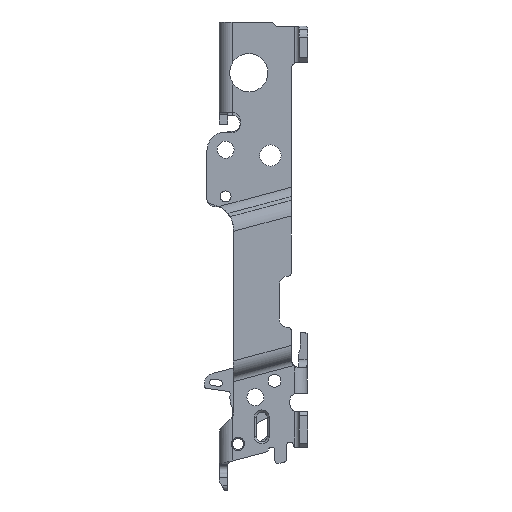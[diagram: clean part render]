
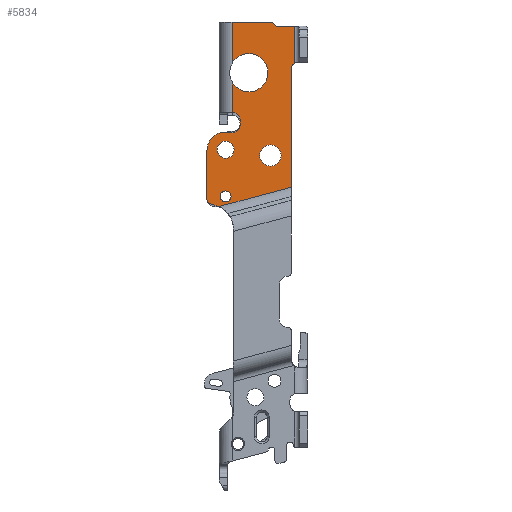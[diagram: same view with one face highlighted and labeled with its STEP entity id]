
A CAD part, left-side view. The second image highlights one B-rep face of the part: STEP entity #5834.
In plain terms, the highlighted planar face has unit normal (-1, 0, 0).
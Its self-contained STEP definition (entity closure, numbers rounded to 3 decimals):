
#43=FACE_BOUND('',#762,.T.);
#44=FACE_BOUND('',#763,.T.);
#45=FACE_BOUND('',#764,.T.);
#209=PLANE('',#6303);
#427=FACE_OUTER_BOUND('',#761,.T.);
#761=EDGE_LOOP('',(#4413,#4414,#4415,#4416,#4417,#4418,#4419,#4420,#4421,
#4422,#4423,#4424,#4425,#4426,#4427,#4428,#4429,#4430,#4431,#4432));
#762=EDGE_LOOP('',(#4433));
#763=EDGE_LOOP('',(#4434));
#764=EDGE_LOOP('',(#4435));
#1129=LINE('',#8839,#1689);
#1133=LINE('',#8849,#1693);
#1139=LINE('',#8872,#1699);
#1140=LINE('',#8874,#1700);
#1215=LINE('',#9234,#1775);
#1237=LINE('',#9377,#1797);
#1238=LINE('',#9381,#1798);
#1239=LINE('',#9384,#1799);
#1240=LINE('',#9386,#1800);
#1241=LINE('',#9388,#1801);
#1242=LINE('',#9390,#1802);
#1243=LINE('',#9392,#1803);
#1244=LINE('',#9393,#1804);
#1689=VECTOR('',#7012,10.);
#1693=VECTOR('',#7024,10.);
#1699=VECTOR('',#7040,10.);
#1700=VECTOR('',#7041,10.);
#1775=VECTOR('',#7314,10.);
#1797=VECTOR('',#7374,10.);
#1798=VECTOR('',#7377,10.);
#1799=VECTOR('',#7380,10.);
#1800=VECTOR('',#7381,10.);
#1801=VECTOR('',#7382,10.);
#1802=VECTOR('',#7383,10.);
#1803=VECTOR('',#7384,10.);
#1804=VECTOR('',#7385,10.);
#2129=CIRCLE('',#6093,2.);
#2173=CIRCLE('',#6180,2.);
#2186=CIRCLE('',#6208,2.);
#2222=CIRCLE('',#6261,2.5);
#2223=CIRCLE('',#6264,1.275);
#2227=CIRCLE('',#6272,4.5);
#2235=CIRCLE('',#6302,1.5);
#2236=CIRCLE('',#6304,4.5);
#2237=CIRCLE('',#6305,1.);
#2238=CIRCLE('',#6306,6.);
#2382=VERTEX_POINT('',#8486);
#2384=VERTEX_POINT('',#8490);
#2385=VERTEX_POINT('',#8494);
#2388=VERTEX_POINT('',#8508);
#2510=VERTEX_POINT('',#8836);
#2511=VERTEX_POINT('',#8838);
#2513=VERTEX_POINT('',#8844);
#2518=VERTEX_POINT('',#8873);
#2534=VERTEX_POINT('',#8996);
#2601=VERTEX_POINT('',#9171);
#2602=VERTEX_POINT('',#9177);
#2610=VERTEX_POINT('',#9231);
#2611=VERTEX_POINT('',#9233);
#2638=VERTEX_POINT('',#9368);
#2640=VERTEX_POINT('',#9374);
#2641=VERTEX_POINT('',#9376);
#2642=VERTEX_POINT('',#9378);
#2643=VERTEX_POINT('',#9380);
#2644=VERTEX_POINT('',#9382);
#2645=VERTEX_POINT('',#9385);
#2646=VERTEX_POINT('',#9387);
#2647=VERTEX_POINT('',#9389);
#2648=VERTEX_POINT('',#9391);
#2960=EDGE_CURVE('',#2382,#2384,#2129,.T.);
#3120=EDGE_CURVE('',#2511,#2510,#1129,.T.);
#3123=EDGE_CURVE('',#2513,#2511,#2173,.T.);
#3126=EDGE_CURVE('',#2384,#2513,#1133,.T.);
#3136=EDGE_CURVE('',#2385,#2382,#1139,.T.);
#3137=EDGE_CURVE('',#2518,#2388,#1140,.T.);
#3166=EDGE_CURVE('',#2534,#2534,#2186,.T.);
#3257=EDGE_CURVE('',#2601,#2601,#2222,.T.);
#3260=EDGE_CURVE('',#2602,#2602,#2223,.T.);
#3267=EDGE_CURVE('',#2388,#2385,#2227,.T.);
#3279=EDGE_CURVE('',#2611,#2610,#1215,.T.);
#3315=EDGE_CURVE('',#2638,#2610,#2235,.T.);
#3317=EDGE_CURVE('',#2510,#2640,#2236,.T.);
#3318=EDGE_CURVE('',#2640,#2641,#1237,.T.);
#3319=EDGE_CURVE('',#2641,#2642,#2237,.T.);
#3320=EDGE_CURVE('',#2642,#2643,#1238,.T.);
#3321=EDGE_CURVE('',#2643,#2644,#2238,.T.);
#3322=EDGE_CURVE('',#2644,#2611,#1239,.T.);
#3323=EDGE_CURVE('',#2645,#2638,#1240,.T.);
#3324=EDGE_CURVE('',#2645,#2646,#1241,.T.);
#3325=EDGE_CURVE('',#2647,#2646,#1242,.T.);
#3326=EDGE_CURVE('',#2647,#2648,#1243,.T.);
#3327=EDGE_CURVE('',#2648,#2518,#1244,.T.);
#4413=ORIENTED_EDGE('',*,*,#3120,.T.);
#4414=ORIENTED_EDGE('',*,*,#3317,.T.);
#4415=ORIENTED_EDGE('',*,*,#3318,.T.);
#4416=ORIENTED_EDGE('',*,*,#3319,.T.);
#4417=ORIENTED_EDGE('',*,*,#3320,.T.);
#4418=ORIENTED_EDGE('',*,*,#3321,.T.);
#4419=ORIENTED_EDGE('',*,*,#3322,.T.);
#4420=ORIENTED_EDGE('',*,*,#3279,.T.);
#4421=ORIENTED_EDGE('',*,*,#3315,.F.);
#4422=ORIENTED_EDGE('',*,*,#3323,.F.);
#4423=ORIENTED_EDGE('',*,*,#3324,.T.);
#4424=ORIENTED_EDGE('',*,*,#3325,.F.);
#4425=ORIENTED_EDGE('',*,*,#3326,.T.);
#4426=ORIENTED_EDGE('',*,*,#3327,.T.);
#4427=ORIENTED_EDGE('',*,*,#3137,.T.);
#4428=ORIENTED_EDGE('',*,*,#3267,.T.);
#4429=ORIENTED_EDGE('',*,*,#3136,.T.);
#4430=ORIENTED_EDGE('',*,*,#2960,.T.);
#4431=ORIENTED_EDGE('',*,*,#3126,.T.);
#4432=ORIENTED_EDGE('',*,*,#3123,.T.);
#4433=ORIENTED_EDGE('',*,*,#3257,.T.);
#4434=ORIENTED_EDGE('',*,*,#3260,.T.);
#4435=ORIENTED_EDGE('',*,*,#3166,.T.);
#5834=ADVANCED_FACE('',(#427,#43,#44,#45),#209,.T.);
#6093=AXIS2_PLACEMENT_3D('',#8492,#6733,#6734);
#6180=AXIS2_PLACEMENT_3D('',#8845,#7018,#7019);
#6208=AXIS2_PLACEMENT_3D('',#8998,#7093,#7094);
#6261=AXIS2_PLACEMENT_3D('',#9173,#7254,#7255);
#6264=AXIS2_PLACEMENT_3D('',#9179,#7262,#7263);
#6272=AXIS2_PLACEMENT_3D('',#9193,#7281,#7282);
#6302=AXIS2_PLACEMENT_3D('',#9371,#7367,#7368);
#6303=AXIS2_PLACEMENT_3D('',#9373,#7370,#7371);
#6304=AXIS2_PLACEMENT_3D('',#9375,#7372,#7373);
#6305=AXIS2_PLACEMENT_3D('',#9379,#7375,#7376);
#6306=AXIS2_PLACEMENT_3D('',#9383,#7378,#7379);
#6733=DIRECTION('center_axis',(1.,0.,0.));
#6734=DIRECTION('ref_axis',(0.,-1.,0.));
#7012=DIRECTION('',(0.,1.,0.));
#7018=DIRECTION('center_axis',(1.,0.,0.));
#7019=DIRECTION('ref_axis',(0.,0.,
-1.));
#7024=DIRECTION('',(0.,0.,-1.));
#7040=DIRECTION('',(0.,0.,-1.));
#7041=DIRECTION('',(0.,0.,-1.));
#7093=DIRECTION('center_axis',(1.,0.,0.));
#7094=DIRECTION('ref_axis',(0.,0.,-1.));
#7254=DIRECTION('center_axis',(1.,0.,0.));
#7255=DIRECTION('ref_axis',(0.,0.,-1.));
#7262=DIRECTION('center_axis',(1.,0.,0.));
#7263=DIRECTION('ref_axis',(0.,0.,-1.));
#7281=DIRECTION('center_axis',(1.,0.,0.));
#7282=DIRECTION('ref_axis',(0.,0.,-1.));
#7314=DIRECTION('',(0.,0.,1.));
#7367=DIRECTION('center_axis',(-1.,0.,0.));
#7368=DIRECTION('ref_axis',(0.,1.,0.));
#7370=DIRECTION('center_axis',(-1.,0.,0.));
#7371=DIRECTION('ref_axis',(0.,-1.,0.));
#7372=DIRECTION('center_axis',(-1.,0.,0.));
#7373=DIRECTION('ref_axis',(0.,0.034,0.999));
#7374=DIRECTION('',(0.,0.,-1.));
#7375=DIRECTION('center_axis',(-1.,0.,0.));
#7376=DIRECTION('ref_axis',(0.,1.,0.));
#7377=DIRECTION('',(0.,-0.966,-0.259));
#7378=DIRECTION('center_axis',(1.,0.,0.));
#7379=DIRECTION('ref_axis',(0.,-1.,0.));
#7380=DIRECTION('',(0.,-0.966,0.259));
#7381=DIRECTION('',(0.,0.,-1.));
#7382=DIRECTION('',(0.,0.,1.));
#7383=DIRECTION('',(0.,-1.,0.));
#7384=DIRECTION('',(0.,0.707,0.707));
#7385=DIRECTION('',(0.,1.,0.));
#8486=CARTESIAN_POINT('',(0.,-1.,88.949));
#8490=CARTESIAN_POINT('',(0.,-2.94,86.95));
#8492=CARTESIAN_POINT('Origin',(0.,-0.94,
86.95));
#8494=CARTESIAN_POINT('',(0.,-1.,96.126));
#8508=CARTESIAN_POINT('',(0.,-1.,100.474));
#8836=CARTESIAN_POINT('',(0.,1.737,84.2));
#8838=CARTESIAN_POINT('',(0.,-0.94,84.2));
#8839=CARTESIAN_POINT('',(0.,3.132,84.2));
#8844=CARTESIAN_POINT('',(0.,-2.94,86.2));
#8845=CARTESIAN_POINT('Origin',(0.,-0.94,
86.2));
#8849=CARTESIAN_POINT('',(0.,-2.94,71.038));
#8872=CARTESIAN_POINT('',(0.,-1.,55.125));
#8873=CARTESIAN_POINT('',(0.,-1.,110.25));
#8874=CARTESIAN_POINT('',(0.,-1.,55.125));
#8996=CARTESIAN_POINT('',(0.,0.51,82.18));
#8998=CARTESIAN_POINT('Origin',(0.,0.51,
80.18));
#9171=CARTESIAN_POINT('',(0.,-10.04,81.3));
#9173=CARTESIAN_POINT('Origin',(0.,-10.04,78.8));
#9177=CARTESIAN_POINT('',(0.,0.51,70.455));
#9179=CARTESIAN_POINT('Origin',(0.,0.51,
69.18));
#9193=CARTESIAN_POINT('Origin',(0.,-4.94,
98.3));
#9231=CARTESIAN_POINT('',(0.,-14.99,99.3));
#9233=CARTESIAN_POINT('',(0.,-14.99,71.342));
#9234=CARTESIAN_POINT('',(0.,-14.99,110.25));
#9368=CARTESIAN_POINT('',(0.,-15.8,100.632));
#9371=CARTESIAN_POINT('Origin',(0.,-16.49,99.3));
#9373=CARTESIAN_POINT('Origin',(0.,7.203,55.125));
#9374=CARTESIAN_POINT('',(0.,4.91,79.9));
#9375=CARTESIAN_POINT('Origin',(0.,0.41,79.9));
#9376=CARTESIAN_POINT('',(0.,4.91,68.376));
#9377=CARTESIAN_POINT('',(0.,4.91,79.9));
#9378=CARTESIAN_POINT('',(0.,4.169,67.41));
#9379=CARTESIAN_POINT('Origin',(0.,3.91,68.376));
#9380=CARTESIAN_POINT('',(0.,3.107,67.126));
#9381=CARTESIAN_POINT('',(0.,4.169,67.41));
#9382=CARTESIAN_POINT('',(0.,2.108,66.76));
#9383=CARTESIAN_POINT('Origin',(0.,4.66,61.33));
#9384=CARTESIAN_POINT('',(0.,13.301,63.761));
#9385=CARTESIAN_POINT('',(0.,-15.8,100.8));
#9386=CARTESIAN_POINT('',(0.,-15.8,27.563));
#9387=CARTESIAN_POINT('',(0.,-15.8,109.3));
#9388=CARTESIAN_POINT('',(0.,-15.8,77.963));
#9389=CARTESIAN_POINT('',(0.,-11.39,109.3));
#9390=CARTESIAN_POINT('',(0.,-14.99,109.3));
#9391=CARTESIAN_POINT('',(0.,-10.44,110.25));
#9392=CARTESIAN_POINT('',(0.,-23.716,96.974));
#9393=CARTESIAN_POINT('',(0.,-1.,110.25));
